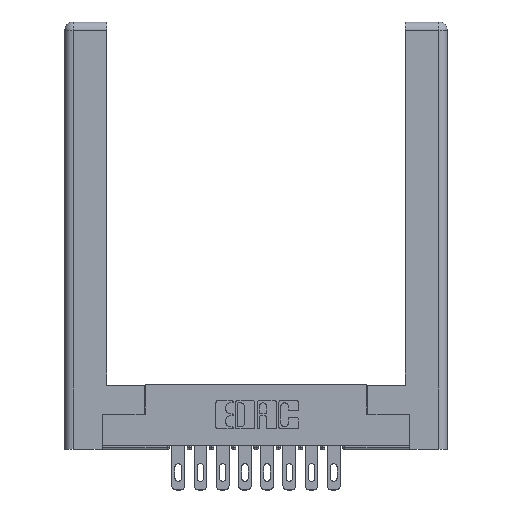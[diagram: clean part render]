
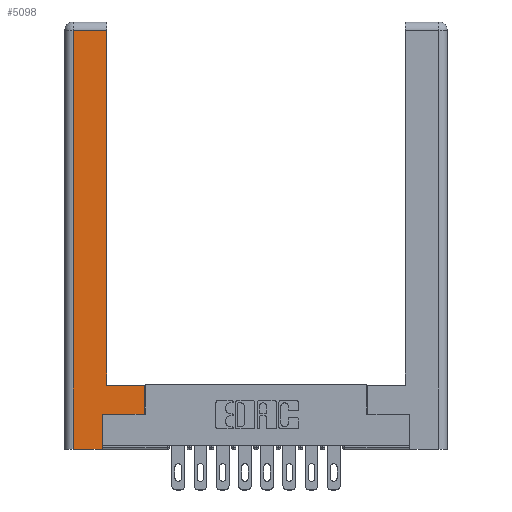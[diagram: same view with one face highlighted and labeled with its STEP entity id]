
A CAD part, top view. The second image highlights one B-rep face of the part: STEP entity #5098.
In plain terms, the highlighted planar face has unit normal (0, 0, 1).
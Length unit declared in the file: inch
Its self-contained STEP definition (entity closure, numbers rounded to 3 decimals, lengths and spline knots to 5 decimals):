
#83 = EDGE_LOOP ( 'NONE', ( #3198, #5319, #5299, #1835, #13327, #9160, #10137, #14189 ) ) ;
#290 = LINE ( 'NONE', #10954, #12423 ) ;
#342 = CARTESIAN_POINT ( 'NONE',  ( 0.295, 3., 0. ) ) ;
#382 = DIRECTION ( 'NONE',  ( -1., 0., 0. ) ) ;
#789 = DIRECTION ( 'NONE',  ( 0., -1., 0. ) ) ;
#919 = DIRECTION ( 'NONE',  ( 0., 1., 0. ) ) ;
#976 = CARTESIAN_POINT ( 'NONE',  ( 0.295, 0.45, 0. ) ) ;
#1038 = VECTOR ( 'NONE', #382, 39.37008 ) ;
#1045 = LINE ( 'NONE', #5530, #9436 ) ;
#1835 = ORIENTED_EDGE ( 'NONE', *, *, #3715, .T. ) ;
#2051 = EDGE_CURVE ( 'NONE', #9776, #9199, #3744, .T. ) ;
#2145 = CARTESIAN_POINT ( 'NONE',  ( 0.565, 0.245, 0. ) ) ;
#3057 = LINE ( 'NONE', #9916, #1038 ) ;
#3198 = ORIENTED_EDGE ( 'NONE', *, *, #6730, .T. ) ;
#3299 = CARTESIAN_POINT ( 'NONE',  ( 0.265, 0., 0. ) ) ;
#3398 = CARTESIAN_POINT ( 'NONE',  ( 0.565, 0.245, 0. ) ) ;
#3715 = EDGE_CURVE ( 'NONE', #6718, #10747, #6333, .T. ) ;
#3744 = LINE ( 'NONE', #3398, #12895 ) ;
#3909 = CARTESIAN_POINT ( 'NONE',  ( 0.565, 0.45, 0. ) ) ;
#3993 = LINE ( 'NONE', #342, #14096 ) ;
#4134 = CARTESIAN_POINT ( 'NONE',  ( 0., 0., 0. ) ) ;
#4175 = EDGE_CURVE ( 'NONE', #7196, #13880, #8005, .T. ) ;
#5098 = ADVANCED_FACE ( 'NONE', ( #8905 ), #7615, .F. ) ;
#5299 = ORIENTED_EDGE ( 'NONE', *, *, #11471, .T. ) ;
#5319 = ORIENTED_EDGE ( 'NONE', *, *, #4175, .T. ) ;
#5530 = CARTESIAN_POINT ( 'NONE',  ( 0.0615, 0., 0. ) ) ;
#6333 = LINE ( 'NONE', #3299, #13453 ) ;
#6718 = VERTEX_POINT ( 'NONE', #10920 ) ;
#6730 = EDGE_CURVE ( 'NONE', #8129, #7196, #3993, .T. ) ;
#6814 = AXIS2_PLACEMENT_3D ( 'NONE', #4134, #13747, #10182 ) ;
#6938 = DIRECTION ( 'NONE',  ( 1., 0., 0. ) ) ;
#7196 = VERTEX_POINT ( 'NONE', #7939 ) ;
#7615 = PLANE ( 'NONE',  #6814 ) ;
#7630 = VECTOR ( 'NONE', #919, 39.37008 ) ;
#7822 = VECTOR ( 'NONE', #14523, 39.37008 ) ;
#7939 = CARTESIAN_POINT ( 'NONE',  ( 0.295, 2.94, 0. ) ) ;
#8005 = LINE ( 'NONE', #15466, #7822 ) ;
#8129 = VERTEX_POINT ( 'NONE', #976 ) ;
#8905 = FACE_OUTER_BOUND ( 'NONE', #83, .T. ) ;
#9160 = ORIENTED_EDGE ( 'NONE', *, *, #2051, .T. ) ;
#9199 = VERTEX_POINT ( 'NONE', #2145 ) ;
#9436 = VECTOR ( 'NONE', #789, 39.37008 ) ;
#9776 = VERTEX_POINT ( 'NONE', #10989 ) ;
#9916 = CARTESIAN_POINT ( 'NONE',  ( 0.295, 0.45, 0. ) ) ;
#10066 = LINE ( 'NONE', #11718, #7630 ) ;
#10137 = ORIENTED_EDGE ( 'NONE', *, *, #14556, .T. ) ;
#10182 = DIRECTION ( 'NONE',  ( -1., 0., 0. ) ) ;
#10747 = VERTEX_POINT ( 'NONE', #13637 ) ;
#10856 = CARTESIAN_POINT ( 'NONE',  ( 0.0615, 2.94, 0. ) ) ;
#10920 = CARTESIAN_POINT ( 'NONE',  ( 0.0615, 0., 0. ) ) ;
#10954 = CARTESIAN_POINT ( 'NONE',  ( 0.565, 0.45, 0. ) ) ;
#10989 = CARTESIAN_POINT ( 'NONE',  ( 0.265, 0.245, 0. ) ) ;
#11022 = DIRECTION ( 'NONE',  ( 0., 1., 0. ) ) ;
#11471 = EDGE_CURVE ( 'NONE', #13880, #6718, #1045, .T. ) ;
#11718 = CARTESIAN_POINT ( 'NONE',  ( 0.265, 0.245, 0. ) ) ;
#11871 = DIRECTION ( 'NONE',  ( 1., 0., 0. ) ) ;
#12158 = DIRECTION ( 'NONE',  ( 0., 1., 0. ) ) ;
#12423 = VECTOR ( 'NONE', #12158, 39.37008 ) ;
#12435 = EDGE_CURVE ( 'NONE', #10747, #9776, #10066, .T. ) ;
#12895 = VECTOR ( 'NONE', #6938, 39.37008 ) ;
#13327 = ORIENTED_EDGE ( 'NONE', *, *, #12435, .T. ) ;
#13453 = VECTOR ( 'NONE', #11871, 39.37008 ) ;
#13637 = CARTESIAN_POINT ( 'NONE',  ( 0.265, 0., 0. ) ) ;
#13747 = DIRECTION ( 'NONE',  ( 0., 0., -1. ) ) ;
#13880 = VERTEX_POINT ( 'NONE', #10856 ) ;
#14096 = VECTOR ( 'NONE', #11022, 39.37008 ) ;
#14189 = ORIENTED_EDGE ( 'NONE', *, *, #14685, .T. ) ;
#14523 = DIRECTION ( 'NONE',  ( -1., 0., 0. ) ) ;
#14556 = EDGE_CURVE ( 'NONE', #9199, #15114, #290, .T. ) ;
#14685 = EDGE_CURVE ( 'NONE', #15114, #8129, #3057, .T. ) ;
#15114 = VERTEX_POINT ( 'NONE', #3909 ) ;
#15466 = CARTESIAN_POINT ( 'NONE',  ( 0.0615, 2.94, 0. ) ) ;
